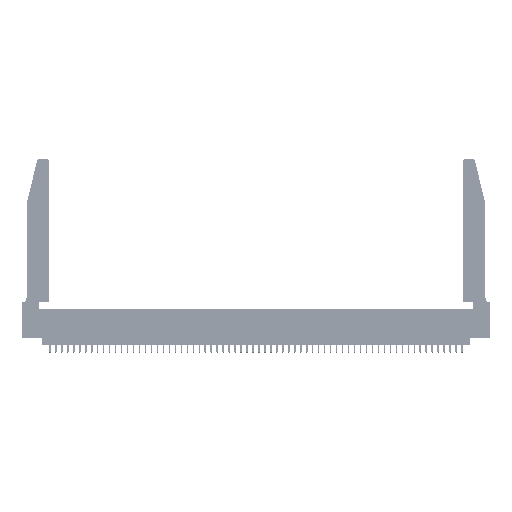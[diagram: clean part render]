
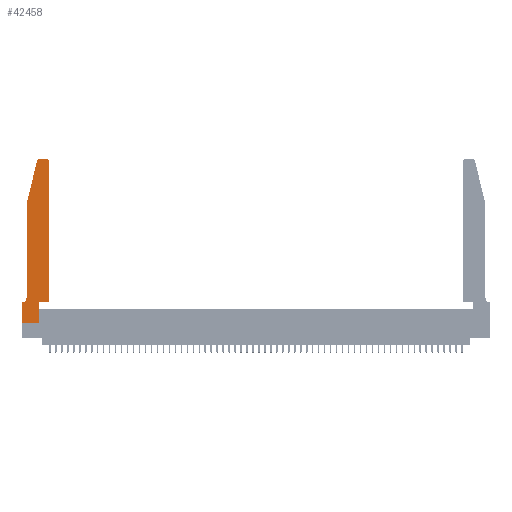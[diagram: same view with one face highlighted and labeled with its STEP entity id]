
A CAD part, top view. The second image highlights one B-rep face of the part: STEP entity #42458.
In plain terms, the highlighted planar face has unit normal (0, 0, 1).
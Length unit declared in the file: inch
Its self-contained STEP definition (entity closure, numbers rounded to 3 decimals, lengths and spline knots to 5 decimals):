
#135 = DIRECTION ( 'NONE',  ( -1., 0., 0. ) ) ;
#370 = VERTEX_POINT ( 'NONE', #44262 ) ;
#683 = EDGE_CURVE ( 'NONE', #4844, #15069, #54318, .T. ) ;
#800 = LINE ( 'NONE', #55272, #32643 ) ;
#1211 = CARTESIAN_POINT ( 'NONE',  ( 0., 0.35, 0.37 ) ) ;
#1399 = CARTESIAN_POINT ( 'NONE',  ( 0.0755, 0.42, 0.37 ) ) ;
#1492 = VECTOR ( 'NONE', #25847, 39.37008 ) ;
#1773 = EDGE_CURVE ( 'NONE', #51000, #4844, #24471, .T. ) ;
#1799 = DIRECTION ( 'NONE',  ( 0., 1., 0. ) ) ;
#2085 = VECTOR ( 'NONE', #31159, 39.37008 ) ;
#3422 = EDGE_CURVE ( 'NONE', #13718, #370, #47472, .T. ) ;
#3540 = CARTESIAN_POINT ( 'NONE',  ( 0.4205, 2.75, 0.37 ) ) ;
#4844 = VERTEX_POINT ( 'NONE', #21856 ) ;
#5153 = EDGE_CURVE ( 'NONE', #370, #25910, #52895, .T. ) ;
#5358 = DIRECTION ( 'NONE',  ( 1., 0., 0. ) ) ;
#6007 = ORIENTED_EDGE ( 'NONE', *, *, #21400, .T. ) ;
#7121 = AXIS2_PLACEMENT_3D ( 'NONE', #12337, #47042, #8171 ) ;
#7402 = CARTESIAN_POINT ( 'NONE',  ( 0.0055, 0.35, 0.37 ) ) ;
#8171 = DIRECTION ( 'NONE',  ( -1., 0., 0. ) ) ;
#8189 = ORIENTED_EDGE ( 'NONE', *, *, #15492, .T. ) ;
#9134 = VERTEX_POINT ( 'NONE', #3540 ) ;
#10987 = LINE ( 'NONE', #47691, #44225 ) ;
#11624 = VECTOR ( 'NONE', #31619, 39.37008 ) ;
#11853 = CARTESIAN_POINT ( 'NONE',  ( 0.25487, 2.72718, 0.37 ) ) ;
#12337 = CARTESIAN_POINT ( 'NONE',  ( 0.0055, 0.42, 0.37 ) ) ;
#13358 = EDGE_CURVE ( 'NONE', #38163, #18037, #40785, .T. ) ;
#13718 = VERTEX_POINT ( 'NONE', #54712 ) ;
#13991 = ORIENTED_EDGE ( 'NONE', *, *, #39826, .T. ) ;
#14053 = PLANE ( 'NONE',  #17197 ) ;
#14839 = EDGE_LOOP ( 'NONE', ( #32582, #26947, #36228, #6007, #52161, #37970, #23034, #22257, #8189, #17351, #34851, #13991 ) ) ;
#15069 = VERTEX_POINT ( 'NONE', #24659 ) ;
#15492 = EDGE_CURVE ( 'NONE', #17564, #13718, #41237, .T. ) ;
#15787 = CIRCLE ( 'NONE', #27301, 0.03 ) ;
#16721 = DIRECTION ( 'NONE',  ( 0., 0., 1. ) ) ;
#17039 = DIRECTION ( 'NONE',  ( 0., -1., 0. ) ) ;
#17197 = AXIS2_PLACEMENT_3D ( 'NONE', #1211, #26960, #5358 ) ;
#17351 = ORIENTED_EDGE ( 'NONE', *, *, #3422, .T. ) ;
#17564 = VERTEX_POINT ( 'NONE', #51516 ) ;
#17792 = CARTESIAN_POINT ( 'NONE',  ( 0.284, 2.75, 0.37 ) ) ;
#18037 = VERTEX_POINT ( 'NONE', #20156 ) ;
#18260 = CARTESIAN_POINT ( 'NONE',  ( 0.284, 2.72, 0.37 ) ) ;
#18697 = DIRECTION ( 'NONE',  ( 0., 1., 0. ) ) ;
#18846 = VERTEX_POINT ( 'NONE', #17792 ) ;
#20156 = CARTESIAN_POINT ( 'NONE',  ( 0.0755, 2., 0.37 ) ) ;
#20913 = DIRECTION ( 'NONE',  ( 1., 0., 0. ) ) ;
#21400 = EDGE_CURVE ( 'NONE', #18037, #49355, #30317, .T. ) ;
#21856 = CARTESIAN_POINT ( 'NONE',  ( 0., 0.35, 0.37 ) ) ;
#22257 = ORIENTED_EDGE ( 'NONE', *, *, #41520, .T. ) ;
#23034 = ORIENTED_EDGE ( 'NONE', *, *, #683, .T. ) ;
#23759 = VECTOR ( 'NONE', #29871, 39.37008 ) ;
#24471 = LINE ( 'NONE', #39861, #2085 ) ;
#24659 = CARTESIAN_POINT ( 'NONE',  ( 0., 0., 0.37 ) ) ;
#24955 = CARTESIAN_POINT ( 'NONE',  ( 0.4505, 0.35, 0.37 ) ) ;
#25234 = EDGE_CURVE ( 'NONE', #9134, #18846, #10987, .T. ) ;
#25291 = CARTESIAN_POINT ( 'NONE',  ( 0., 0., 0.37 ) ) ;
#25418 = CIRCLE ( 'NONE', #32564, 0.03 ) ;
#25847 = DIRECTION ( 'NONE',  ( 0., -1., 0. ) ) ;
#25910 = VERTEX_POINT ( 'NONE', #31879 ) ;
#26267 = DIRECTION ( 'NONE',  ( 1., 0., 0. ) ) ;
#26288 = FACE_OUTER_BOUND ( 'NONE', #14839, .T. ) ;
#26947 = ORIENTED_EDGE ( 'NONE', *, *, #34887, .T. ) ;
#26960 = DIRECTION ( 'NONE',  ( 0., 0., 1. ) ) ;
#27301 = AXIS2_PLACEMENT_3D ( 'NONE', #51619, #16721, #47460 ) ;
#27633 = CARTESIAN_POINT ( 'NONE',  ( 0.2865, 0.35, 0.37 ) ) ;
#29871 = DIRECTION ( 'NONE',  ( 1., 0., 0. ) ) ;
#30317 = LINE ( 'NONE', #42850, #52004 ) ;
#31159 = DIRECTION ( 'NONE',  ( -1., 0., 0. ) ) ;
#31619 = DIRECTION ( 'NONE',  ( -0.239, -0.971, 0. ) ) ;
#31879 = CARTESIAN_POINT ( 'NONE',  ( 0.4505, 2.72, 0.37 ) ) ;
#32564 = AXIS2_PLACEMENT_3D ( 'NONE', #18260, #52562, #26267 ) ;
#32582 = ORIENTED_EDGE ( 'NONE', *, *, #25234, .T. ) ;
#32643 = VECTOR ( 'NONE', #20913, 39.37008 ) ;
#34851 = ORIENTED_EDGE ( 'NONE', *, *, #5153, .T. ) ;
#34887 = EDGE_CURVE ( 'NONE', #18846, #38163, #25418, .T. ) ;
#36228 = ORIENTED_EDGE ( 'NONE', *, *, #13358, .T. ) ;
#36814 = CARTESIAN_POINT ( 'NONE',  ( 0.4505, 0.35, 0.37 ) ) ;
#37970 = ORIENTED_EDGE ( 'NONE', *, *, #1773, .T. ) ;
#38163 = VERTEX_POINT ( 'NONE', #11853 ) ;
#39826 = EDGE_CURVE ( 'NONE', #25910, #9134, #15787, .T. ) ;
#39861 = CARTESIAN_POINT ( 'NONE',  ( 0.0755, 0.35, 0.37 ) ) ;
#40785 = LINE ( 'NONE', #45095, #11624 ) ;
#41237 = LINE ( 'NONE', #27633, #50075 ) ;
#41520 = EDGE_CURVE ( 'NONE', #15069, #17564, #800, .T. ) ;
#42104 = VECTOR ( 'NONE', #1799, 39.37008 ) ;
#42458 = ADVANCED_FACE ( 'NONE', ( #26288 ), #14053, .T. ) ;
#42850 = CARTESIAN_POINT ( 'NONE',  ( 0.0755, 2., 0.37 ) ) ;
#44225 = VECTOR ( 'NONE', #135, 39.37008 ) ;
#44262 = CARTESIAN_POINT ( 'NONE',  ( 0.4505, 0.35, 0.37 ) ) ;
#45095 = CARTESIAN_POINT ( 'NONE',  ( 0.0755, 2., 0.37 ) ) ;
#47042 = DIRECTION ( 'NONE',  ( 0., 0., -1. ) ) ;
#47460 = DIRECTION ( 'NONE',  ( 1., 0., 0. ) ) ;
#47472 = LINE ( 'NONE', #24955, #23759 ) ;
#47691 = CARTESIAN_POINT ( 'NONE',  ( 0.2605, 2.75, 0.37 ) ) ;
#49355 = VERTEX_POINT ( 'NONE', #1399 ) ;
#50075 = VECTOR ( 'NONE', #18697, 39.37008 ) ;
#51000 = VERTEX_POINT ( 'NONE', #7402 ) ;
#51159 = CIRCLE ( 'NONE', #7121, 0.07 ) ;
#51516 = CARTESIAN_POINT ( 'NONE',  ( 0.2865, 0., 0.37 ) ) ;
#51619 = CARTESIAN_POINT ( 'NONE',  ( 0.4205, 2.72, 0.37 ) ) ;
#52004 = VECTOR ( 'NONE', #17039, 39.37008 ) ;
#52161 = ORIENTED_EDGE ( 'NONE', *, *, #54226, .T. ) ;
#52562 = DIRECTION ( 'NONE',  ( 0., 0., 1. ) ) ;
#52895 = LINE ( 'NONE', #36814, #42104 ) ;
#54226 = EDGE_CURVE ( 'NONE', #49355, #51000, #51159, .T. ) ;
#54318 = LINE ( 'NONE', #25291, #1492 ) ;
#54712 = CARTESIAN_POINT ( 'NONE',  ( 0.2865, 0.35, 0.37 ) ) ;
#55272 = CARTESIAN_POINT ( 'NONE',  ( 0., 0., 0.37 ) ) ;
